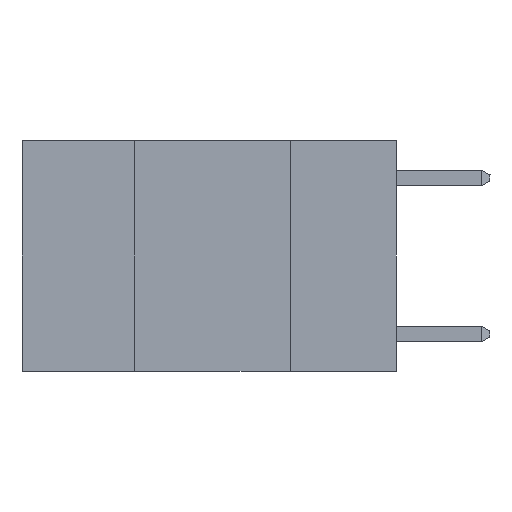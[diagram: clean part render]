
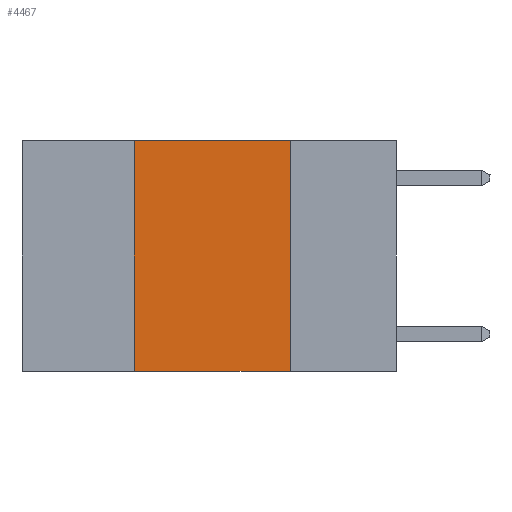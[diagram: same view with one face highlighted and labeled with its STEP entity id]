
A CAD part, left-side view. The second image highlights one B-rep face of the part: STEP entity #4467.
In plain terms, the highlighted planar face has unit normal (-1, 0, 0).
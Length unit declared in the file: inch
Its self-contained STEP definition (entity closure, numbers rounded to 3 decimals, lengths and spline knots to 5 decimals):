
#598 = VECTOR ( 'NONE', #3491, 39.37008 ) ;
#660 = DIRECTION ( 'NONE',  ( 0., -1., 0. ) ) ;
#1487 = DIRECTION ( 'NONE',  ( 1., 0., 0. ) ) ;
#1516 = LINE ( 'NONE', #8415, #10306 ) ;
#1790 = VECTOR ( 'NONE', #10058, 39.37008 ) ;
#2244 = CARTESIAN_POINT ( 'NONE',  ( 0., 0.6, 0. ) ) ;
#2660 = CARTESIAN_POINT ( 'NONE',  ( 0., 0.17, 0. ) ) ;
#2725 = CARTESIAN_POINT ( 'NONE',  ( 0., 0.17, 0. ) ) ;
#2759 = ORIENTED_EDGE ( 'NONE', *, *, #5886, .T. ) ;
#2761 = EDGE_CURVE ( 'NONE', #7283, #7741, #10532, .T. ) ;
#2832 = LINE ( 'NONE', #2725, #598 ) ;
#3340 = LINE ( 'NONE', #8241, #1790 ) ;
#3491 = DIRECTION ( 'NONE',  ( 0., 0., -1. ) ) ;
#3858 = CARTESIAN_POINT ( 'NONE',  ( 0., 0.17, -0.37 ) ) ;
#4089 = PLANE ( 'NONE',  #9536 ) ;
#4467 = ADVANCED_FACE ( 'NONE', ( #6573 ), #4089, .F. ) ;
#5294 = VERTEX_POINT ( 'NONE', #3858 ) ;
#5456 = EDGE_CURVE ( 'NONE', #10492, #7283, #3340, .T. ) ;
#5886 = EDGE_CURVE ( 'NONE', #10492, #5294, #1516, .T. ) ;
#6155 = ORIENTED_EDGE ( 'NONE', *, *, #5456, .F. ) ;
#6573 = FACE_OUTER_BOUND ( 'NONE', #8028, .T. ) ;
#7283 = VERTEX_POINT ( 'NONE', #8687 ) ;
#7437 = DIRECTION ( 'NONE',  ( 0., -1., 0. ) ) ;
#7661 = CARTESIAN_POINT ( 'NONE',  ( 0., 0.6, 0. ) ) ;
#7741 = VERTEX_POINT ( 'NONE', #2660 ) ;
#8028 = EDGE_LOOP ( 'NONE', ( #10739, #10664, #6155, #2759 ) ) ;
#8241 = CARTESIAN_POINT ( 'NONE',  ( 0., 0.42, 0. ) ) ;
#8415 = CARTESIAN_POINT ( 'NONE',  ( 0., 0.6, -0.37 ) ) ;
#8687 = CARTESIAN_POINT ( 'NONE',  ( 0., 0.42, 0. ) ) ;
#9140 = CARTESIAN_POINT ( 'NONE',  ( 0., 0.42, -0.37 ) ) ;
#9147 = DIRECTION ( 'NONE',  ( 0., 0., -1. ) ) ;
#9222 = VECTOR ( 'NONE', #7437, 39.37008 ) ;
#9536 = AXIS2_PLACEMENT_3D ( 'NONE', #7661, #1487, #9147 ) ;
#10058 = DIRECTION ( 'NONE',  ( 0., 0., 1. ) ) ;
#10306 = VECTOR ( 'NONE', #660, 39.37008 ) ;
#10492 = VERTEX_POINT ( 'NONE', #9140 ) ;
#10532 = LINE ( 'NONE', #2244, #9222 ) ;
#10664 = ORIENTED_EDGE ( 'NONE', *, *, #2761, .F. ) ;
#10739 = ORIENTED_EDGE ( 'NONE', *, *, #11138, .F. ) ;
#11138 = EDGE_CURVE ( 'NONE', #7741, #5294, #2832, .T. ) ;
